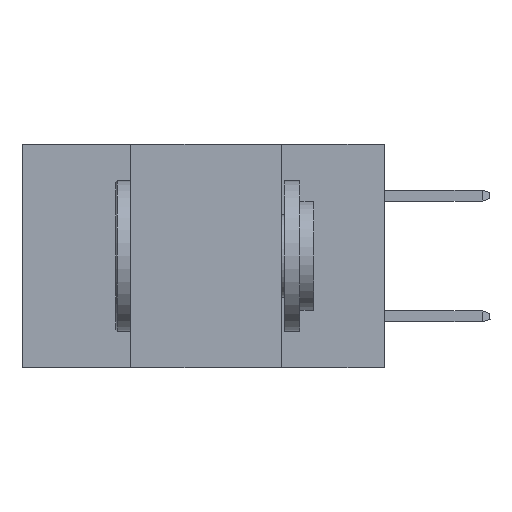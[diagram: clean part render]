
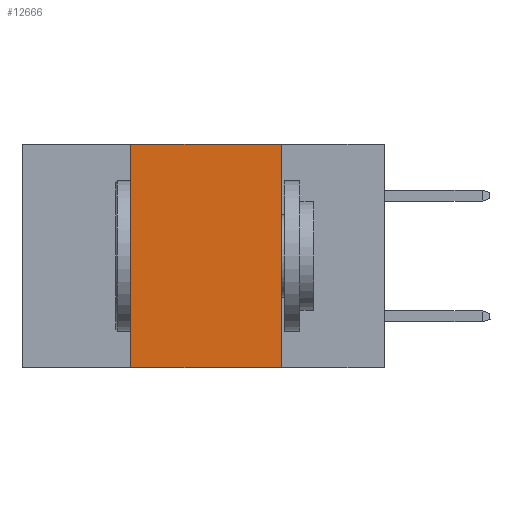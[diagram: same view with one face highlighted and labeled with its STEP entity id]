
A CAD part, left-side view. The second image highlights one B-rep face of the part: STEP entity #12666.
In plain terms, the highlighted planar face has unit normal (-1, 0, 0).
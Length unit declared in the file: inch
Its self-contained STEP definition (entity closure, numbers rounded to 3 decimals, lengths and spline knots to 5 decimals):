
#478 = ORIENTED_EDGE ( 'NONE', *, *, #17606, .F. ) ;
#761 = AXIS2_PLACEMENT_3D ( 'NONE', #8921, #19699, #10482 ) ;
#968 = CARTESIAN_POINT ( 'NONE',  ( 0., 0.6, -0.37 ) ) ;
#2265 = CARTESIAN_POINT ( 'NONE',  ( 0., 0.42, -0.37 ) ) ;
#3254 = VERTEX_POINT ( 'NONE', #16252 ) ;
#4215 = DIRECTION ( 'NONE',  ( 0., -1., 0. ) ) ;
#5277 = ORIENTED_EDGE ( 'NONE', *, *, #15650, .T. ) ;
#5324 = EDGE_CURVE ( 'NONE', #18736, #7399, #19614, .T. ) ;
#5816 = PLANE ( 'NONE',  #761 ) ;
#5844 = CARTESIAN_POINT ( 'NONE',  ( 0., 0.17, -0.37 ) ) ;
#7399 = VERTEX_POINT ( 'NONE', #5844 ) ;
#8905 = FACE_OUTER_BOUND ( 'NONE', #16057, .T. ) ;
#8921 = CARTESIAN_POINT ( 'NONE',  ( 0., 0.6, 0. ) ) ;
#9451 = LINE ( 'NONE', #12568, #12617 ) ;
#10075 = VERTEX_POINT ( 'NONE', #2265 ) ;
#10179 = CARTESIAN_POINT ( 'NONE',  ( 0., 0.17, 0. ) ) ;
#10482 = DIRECTION ( 'NONE',  ( 0., 0., -1. ) ) ;
#10889 = EDGE_CURVE ( 'NONE', #3254, #18736, #9451, .T. ) ;
#11103 = ORIENTED_EDGE ( 'NONE', *, *, #10889, .F. ) ;
#12250 = VECTOR ( 'NONE', #4215, 39.37008 ) ;
#12401 = VECTOR ( 'NONE', #18378, 39.37008 ) ;
#12568 = CARTESIAN_POINT ( 'NONE',  ( 0., 0.6, 0. ) ) ;
#12617 = VECTOR ( 'NONE', #18761, 39.37008 ) ;
#12666 = ADVANCED_FACE ( 'NONE', ( #8905 ), #5816, .F. ) ;
#13376 = LINE ( 'NONE', #19901, #12401 ) ;
#13577 = DIRECTION ( 'NONE',  ( 0., 0., -1. ) ) ;
#13642 = CARTESIAN_POINT ( 'NONE',  ( 0., 0.17, -0.37 ) ) ;
#15568 = VECTOR ( 'NONE', #13577, 39.37008 ) ;
#15650 = EDGE_CURVE ( 'NONE', #10075, #7399, #16375, .T. ) ;
#16057 = EDGE_LOOP ( 'NONE', ( #18808, #11103, #478, #5277 ) ) ;
#16252 = CARTESIAN_POINT ( 'NONE',  ( 0., 0.42, 0. ) ) ;
#16375 = LINE ( 'NONE', #968, #12250 ) ;
#17606 = EDGE_CURVE ( 'NONE', #10075, #3254, #13376, .T. ) ;
#18378 = DIRECTION ( 'NONE',  ( 0., 0., 1. ) ) ;
#18736 = VERTEX_POINT ( 'NONE', #10179 ) ;
#18761 = DIRECTION ( 'NONE',  ( 0., -1., 0. ) ) ;
#18808 = ORIENTED_EDGE ( 'NONE', *, *, #5324, .F. ) ;
#19614 = LINE ( 'NONE', #13642, #15568 ) ;
#19699 = DIRECTION ( 'NONE',  ( 1., 0., 0. ) ) ;
#19901 = CARTESIAN_POINT ( 'NONE',  ( 0., 0.42, -0.37 ) ) ;
